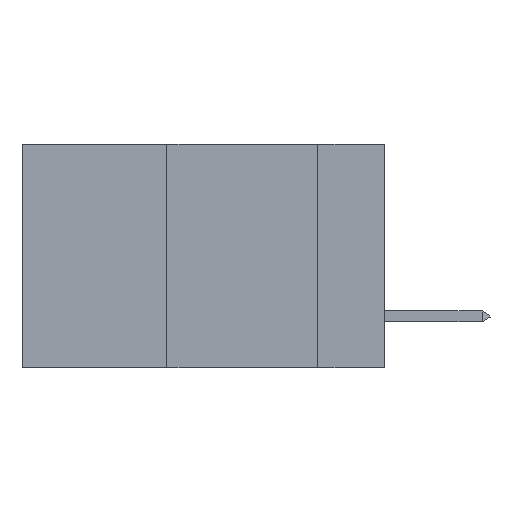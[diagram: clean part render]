
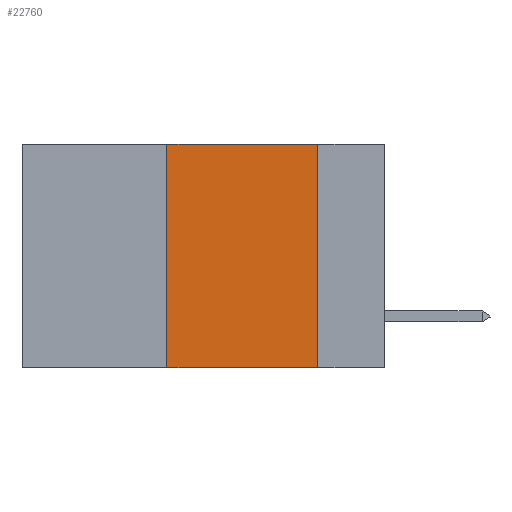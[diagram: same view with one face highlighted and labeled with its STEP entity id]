
A CAD part, left-side view. The second image highlights one B-rep face of the part: STEP entity #22760.
In plain terms, the highlighted planar face has unit normal (-1, 0, 0).
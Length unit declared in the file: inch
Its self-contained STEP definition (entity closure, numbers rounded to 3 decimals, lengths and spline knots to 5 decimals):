
#78 = EDGE_CURVE ( 'NONE', #7015, #20785, #24366, .T. ) ;
#222 = LINE ( 'NONE', #10180, #873 ) ;
#677 = AXIS2_PLACEMENT_3D ( 'NONE', #20698, #18956, #6294 ) ;
#799 = CARTESIAN_POINT ( 'NONE',  ( 0., 0.36, 0. ) ) ;
#873 = VECTOR ( 'NONE', #20332, 39.37008 ) ;
#1869 = LINE ( 'NONE', #799, #11955 ) ;
#2262 = VECTOR ( 'NONE', #23478, 39.37008 ) ;
#2355 = PLANE ( 'NONE',  #677 ) ;
#4028 = VECTOR ( 'NONE', #11285, 39.37008 ) ;
#5651 = CARTESIAN_POINT ( 'NONE',  ( 0., 0.11, 0. ) ) ;
#6294 = DIRECTION ( 'NONE',  ( 0., 0., -1. ) ) ;
#7015 = VERTEX_POINT ( 'NONE', #5651 ) ;
#7753 = VERTEX_POINT ( 'NONE', #11890 ) ;
#9570 = LINE ( 'NONE', #13641, #4028 ) ;
#10180 = CARTESIAN_POINT ( 'NONE',  ( 0., 0.6, -0.37 ) ) ;
#10340 = FACE_OUTER_BOUND ( 'NONE', #17977, .T. ) ;
#10374 = ORIENTED_EDGE ( 'NONE', *, *, #16879, .F. ) ;
#10635 = CARTESIAN_POINT ( 'NONE',  ( 0., 0.36, 0. ) ) ;
#11285 = DIRECTION ( 'NONE',  ( 0., -1., 0. ) ) ;
#11513 = EDGE_CURVE ( 'NONE', #7753, #20785, #222, .T. ) ;
#11666 = ORIENTED_EDGE ( 'NONE', *, *, #11513, .T. ) ;
#11890 = CARTESIAN_POINT ( 'NONE',  ( 0., 0.36, -0.37 ) ) ;
#11955 = VECTOR ( 'NONE', #13341, 39.37008 ) ;
#12567 = CARTESIAN_POINT ( 'NONE',  ( 0., 0.11, -0.37 ) ) ;
#13341 = DIRECTION ( 'NONE',  ( 0., 0., 1. ) ) ;
#13641 = CARTESIAN_POINT ( 'NONE',  ( 0., 0.6, 0. ) ) ;
#16879 = EDGE_CURVE ( 'NONE', #7753, #19779, #1869, .T. ) ;
#17977 = EDGE_LOOP ( 'NONE', ( #19606, #18745, #10374, #11666 ) ) ;
#18745 = ORIENTED_EDGE ( 'NONE', *, *, #25334, .F. ) ;
#18956 = DIRECTION ( 'NONE',  ( 1., 0., 0. ) ) ;
#19375 = CARTESIAN_POINT ( 'NONE',  ( 0., 0.11, 0. ) ) ;
#19606 = ORIENTED_EDGE ( 'NONE', *, *, #78, .F. ) ;
#19779 = VERTEX_POINT ( 'NONE', #10635 ) ;
#20332 = DIRECTION ( 'NONE',  ( 0., -1., 0. ) ) ;
#20698 = CARTESIAN_POINT ( 'NONE',  ( 0., 0.6, 0. ) ) ;
#20785 = VERTEX_POINT ( 'NONE', #12567 ) ;
#22760 = ADVANCED_FACE ( 'NONE', ( #10340 ), #2355, .F. ) ;
#23478 = DIRECTION ( 'NONE',  ( 0., 0., -1. ) ) ;
#24366 = LINE ( 'NONE', #19375, #2262 ) ;
#25334 = EDGE_CURVE ( 'NONE', #19779, #7015, #9570, .T. ) ;
